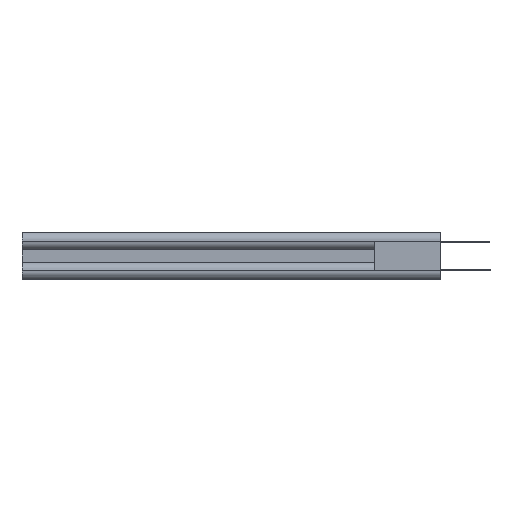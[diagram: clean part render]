
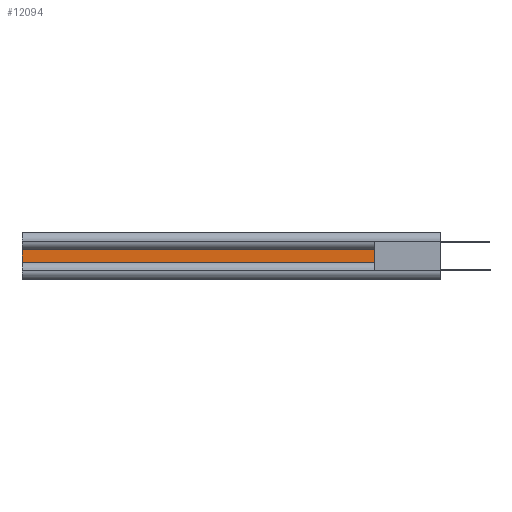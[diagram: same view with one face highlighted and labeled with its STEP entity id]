
A CAD part, left-side view. The second image highlights one B-rep face of the part: STEP entity #12094.
In plain terms, the highlighted planar face has unit normal (-1, 0, 0).
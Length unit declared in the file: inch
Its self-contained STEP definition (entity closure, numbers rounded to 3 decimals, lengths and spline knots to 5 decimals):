
#1000 = VERTEX_POINT ( 'NONE', #4555 ) ;
#1559 = DIRECTION ( 'NONE',  ( 0., 0., -1. ) ) ;
#1563 = ORIENTED_EDGE ( 'NONE', *, *, #2003, .F. ) ;
#1855 = DIRECTION ( 'NONE',  ( 0., 1., 0. ) ) ;
#2003 = EDGE_CURVE ( 'NONE', #16266, #16748, #16517, .T. ) ;
#2032 = ORIENTED_EDGE ( 'NONE', *, *, #13373, .T. ) ;
#2171 = DIRECTION ( 'NONE',  ( 0., 1., 0. ) ) ;
#2461 = VECTOR ( 'NONE', #12069, 39.37008 ) ;
#4179 = ORIENTED_EDGE ( 'NONE', *, *, #5397, .F. ) ;
#4555 = CARTESIAN_POINT ( 'NONE',  ( 0.044, 3., 0.0465 ) ) ;
#4718 = VECTOR ( 'NONE', #2171, 39.37008 ) ;
#5390 = VECTOR ( 'NONE', #19796, 39.37008 ) ;
#5397 = EDGE_CURVE ( 'NONE', #16748, #6079, #21894, .T. ) ;
#5639 = CARTESIAN_POINT ( 'NONE',  ( 0.044, 0.37012, -0.0465 ) ) ;
#6079 = VERTEX_POINT ( 'NONE', #17661 ) ;
#6948 = FACE_OUTER_BOUND ( 'NONE', #18512, .T. ) ;
#8749 = CARTESIAN_POINT ( 'NONE',  ( 0.044, 0.37012, 0.0465 ) ) ;
#9907 = CARTESIAN_POINT ( 'NONE',  ( 0.044, 3., -0.0465 ) ) ;
#10108 = CARTESIAN_POINT ( 'NONE',  ( 0.044, 0.37012, -0.0465 ) ) ;
#11348 = EDGE_CURVE ( 'NONE', #1000, #6079, #18239, .T. ) ;
#11889 = DIRECTION ( 'NONE',  ( 1., 0., 0. ) ) ;
#12069 = DIRECTION ( 'NONE',  ( 0., 0., -1. ) ) ;
#12094 = ADVANCED_FACE ( 'NONE', ( #6948 ), #20056, .F. ) ;
#13256 = CARTESIAN_POINT ( 'NONE',  ( 0.044, 0.473, -0.0465 ) ) ;
#13373 = EDGE_CURVE ( 'NONE', #16266, #1000, #14311, .T. ) ;
#13426 = AXIS2_PLACEMENT_3D ( 'NONE', #10108, #11889, #1559 ) ;
#13805 = VECTOR ( 'NONE', #1855, 39.37008 ) ;
#14311 = LINE ( 'NONE', #8749, #13805 ) ;
#14821 = ORIENTED_EDGE ( 'NONE', *, *, #11348, .T. ) ;
#15529 = CARTESIAN_POINT ( 'NONE',  ( 0.044, 0.473, 0.0465 ) ) ;
#16266 = VERTEX_POINT ( 'NONE', #15529 ) ;
#16517 = LINE ( 'NONE', #13256, #2461 ) ;
#16748 = VERTEX_POINT ( 'NONE', #17588 ) ;
#17588 = CARTESIAN_POINT ( 'NONE',  ( 0.044, 0.473, -0.0465 ) ) ;
#17661 = CARTESIAN_POINT ( 'NONE',  ( 0.044, 3., -0.0465 ) ) ;
#18239 = LINE ( 'NONE', #9907, #5390 ) ;
#18512 = EDGE_LOOP ( 'NONE', ( #2032, #14821, #4179, #1563 ) ) ;
#19796 = DIRECTION ( 'NONE',  ( 0., 0., -1. ) ) ;
#20056 = PLANE ( 'NONE',  #13426 ) ;
#21894 = LINE ( 'NONE', #5639, #4718 ) ;
